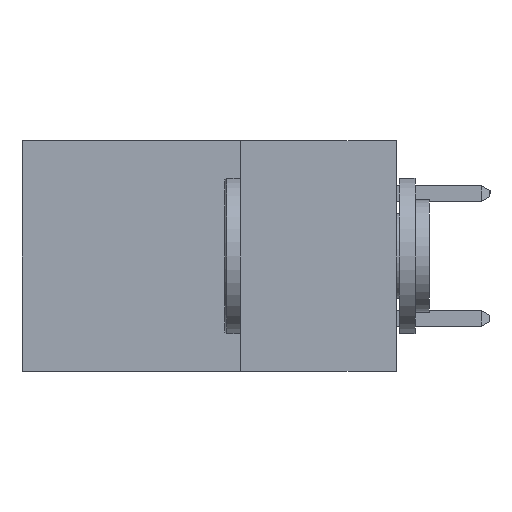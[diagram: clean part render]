
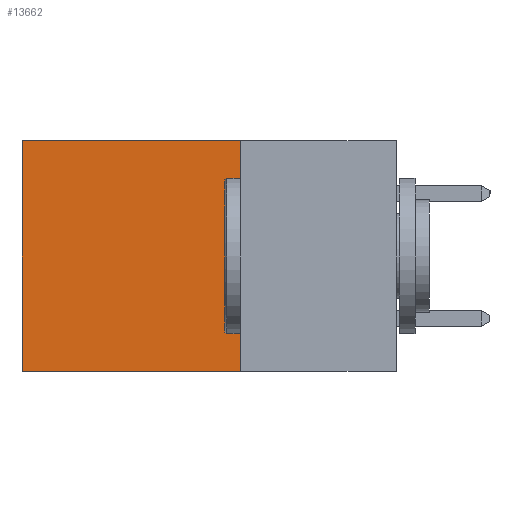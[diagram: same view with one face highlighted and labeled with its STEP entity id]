
A CAD part, left-side view. The second image highlights one B-rep face of the part: STEP entity #13662.
In plain terms, the highlighted planar face has unit normal (-1, 0, 0).
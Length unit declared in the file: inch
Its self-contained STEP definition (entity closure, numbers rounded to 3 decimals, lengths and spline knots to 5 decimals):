
#414 = ORIENTED_EDGE ( 'NONE', *, *, #15301, .F. ) ;
#468 = CARTESIAN_POINT ( 'NONE',  ( 0.2615, 0.25, 0. ) ) ;
#744 = FACE_OUTER_BOUND ( 'NONE', #2356, .T. ) ;
#948 = DIRECTION ( 'NONE',  ( 0., 0., -1. ) ) ;
#1114 = ORIENTED_EDGE ( 'NONE', *, *, #11633, .T. ) ;
#2059 = CARTESIAN_POINT ( 'NONE',  ( 0.2615, 0.6, -0.37 ) ) ;
#2356 = EDGE_LOOP ( 'NONE', ( #4586, #14475, #414, #1114 ) ) ;
#2910 = DIRECTION ( 'NONE',  ( 0., 1., 0. ) ) ;
#3765 = LINE ( 'NONE', #11994, #15847 ) ;
#4176 = DIRECTION ( 'NONE',  ( 0., 0., -1. ) ) ;
#4586 = ORIENTED_EDGE ( 'NONE', *, *, #18181, .T. ) ;
#5724 = CARTESIAN_POINT ( 'NONE',  ( 0.2615, 0.25, -0.37 ) ) ;
#5895 = LINE ( 'NONE', #14677, #9998 ) ;
#6162 = CARTESIAN_POINT ( 'NONE',  ( 0.2615, 0.25, -0.37 ) ) ;
#7946 = AXIS2_PLACEMENT_3D ( 'NONE', #12340, #14305, #948 ) ;
#9678 = CARTESIAN_POINT ( 'NONE',  ( 0.2615, 0.25, 0. ) ) ;
#9998 = VECTOR ( 'NONE', #4176, 39.37008 ) ;
#11633 = EDGE_CURVE ( 'NONE', #13749, #21294, #15455, .T. ) ;
#11994 = CARTESIAN_POINT ( 'NONE',  ( 0.2615, 0.25, -0.37 ) ) ;
#12340 = CARTESIAN_POINT ( 'NONE',  ( 0.2615, 0.25, -0.37 ) ) ;
#12446 = PLANE ( 'NONE',  #7946 ) ;
#12672 = LINE ( 'NONE', #6162, #18393 ) ;
#13662 = ADVANCED_FACE ( 'NONE', ( #744 ), #12446, .F. ) ;
#13749 = VERTEX_POINT ( 'NONE', #9678 ) ;
#13847 = DIRECTION ( 'NONE',  ( 0., 0., -1. ) ) ;
#14305 = DIRECTION ( 'NONE',  ( 1., 0., 0. ) ) ;
#14475 = ORIENTED_EDGE ( 'NONE', *, *, #20439, .F. ) ;
#14677 = CARTESIAN_POINT ( 'NONE',  ( 0.2615, 0.6, -0.37 ) ) ;
#14854 = VERTEX_POINT ( 'NONE', #2059 ) ;
#14898 = VECTOR ( 'NONE', #20445, 39.37008 ) ;
#15301 = EDGE_CURVE ( 'NONE', #13749, #20536, #3765, .T. ) ;
#15455 = LINE ( 'NONE', #468, #14898 ) ;
#15847 = VECTOR ( 'NONE', #13847, 39.37008 ) ;
#18181 = EDGE_CURVE ( 'NONE', #21294, #14854, #5895, .T. ) ;
#18393 = VECTOR ( 'NONE', #2910, 39.37008 ) ;
#20129 = CARTESIAN_POINT ( 'NONE',  ( 0.2615, 0.6, 0. ) ) ;
#20439 = EDGE_CURVE ( 'NONE', #20536, #14854, #12672, .T. ) ;
#20445 = DIRECTION ( 'NONE',  ( 0., 1., 0. ) ) ;
#20536 = VERTEX_POINT ( 'NONE', #5724 ) ;
#21294 = VERTEX_POINT ( 'NONE', #20129 ) ;
